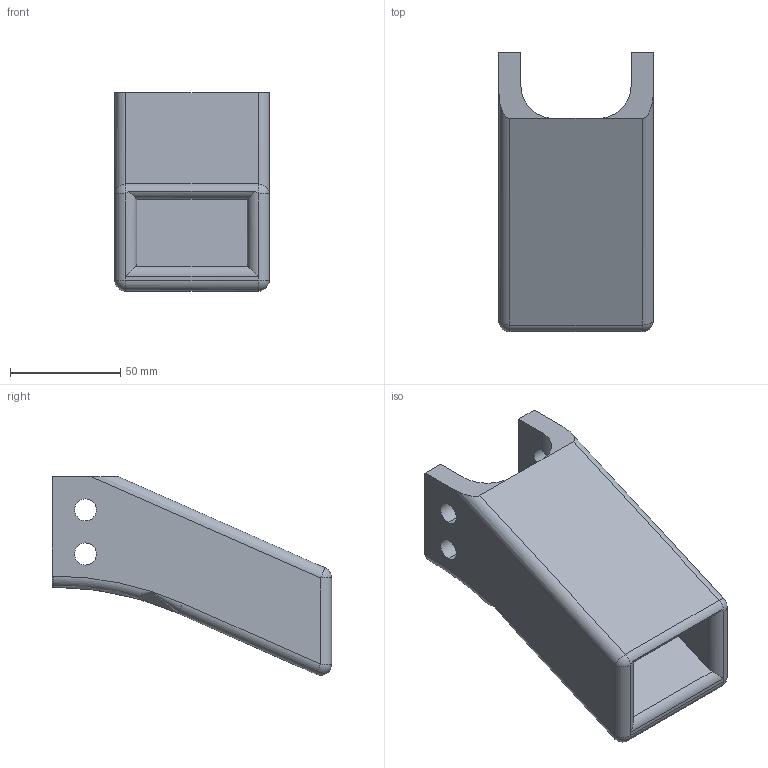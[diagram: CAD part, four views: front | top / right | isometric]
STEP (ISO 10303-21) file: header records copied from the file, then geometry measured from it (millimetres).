
FILE_DESCRIPTION (( 'STEP AP203' ), '1' );
FILE_NAME ('Handle.STEP', '2013-08-23T03:57:39', ( '' ), ( '' ), 'SwSTEP 2.0', 'SolidWorks 2013', '' );
FILE_SCHEMA (( 'CONFIG_CONTROL_DESIGN' ));
Length unit declared in the file: millimetre
Products named in the file (1): Handle
Bounding box: 70 x 126.54 x 89.93 mm (x, y, z)
Volume: 232706.4 mm3; surface area: 52140.7 mm2
Topology: 1 solids, 1 shells, 55 faces, 144 edges, 81 vertices
Faces by surface type: cylinder 27, plane 19, sphere 5, torus 2, bspline 2
Entity records: 1943 total; most frequent: CARTESIAN_POINT 571, ORIENTED_EDGE 276, DIRECTION 270, EDGE_CURVE 138, AXIS2_PLACEMENT_3D 98, VERTEX_POINT 81, VECTOR 74, LINE 74
